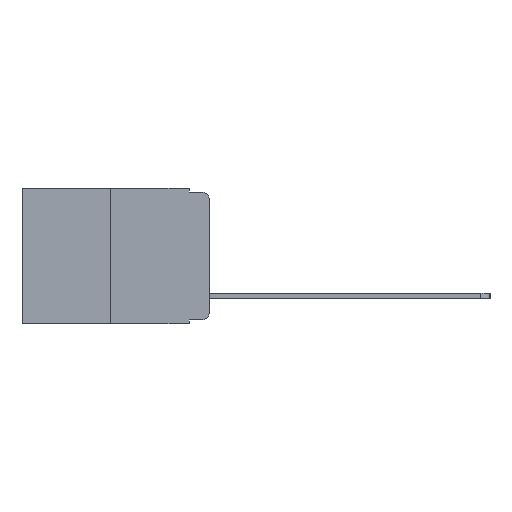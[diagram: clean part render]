
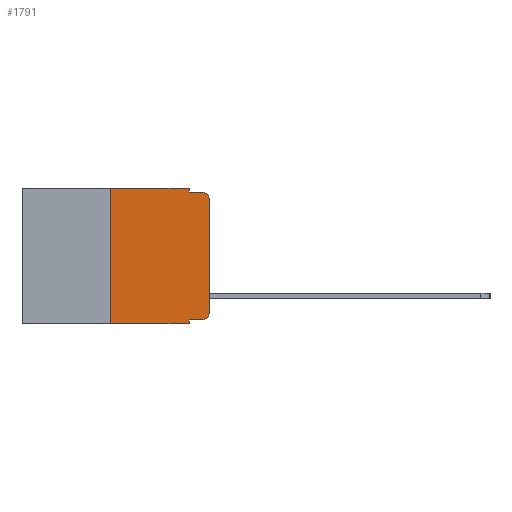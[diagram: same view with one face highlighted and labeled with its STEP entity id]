
A CAD part, left-side view. The second image highlights one B-rep face of the part: STEP entity #1791.
In plain terms, the highlighted planar face has unit normal (-1, 0, 0).
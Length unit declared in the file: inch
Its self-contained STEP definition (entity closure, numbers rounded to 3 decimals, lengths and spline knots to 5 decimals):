
#466 = ORIENTED_EDGE ( 'NONE', *, *, #8201, .T. ) ;
#548 = VERTEX_POINT ( 'NONE', #7839 ) ;
#556 = ORIENTED_EDGE ( 'NONE', *, *, #7493, .F. ) ;
#590 = EDGE_CURVE ( 'NONE', #3171, #14071, #6019, .T. ) ;
#1048 = DIRECTION ( 'NONE',  ( 0., 0., -1. ) ) ;
#1083 = CARTESIAN_POINT ( 'NONE',  ( 0., 0.25, 0. ) ) ;
#1155 = ORIENTED_EDGE ( 'NONE', *, *, #3099, .F. ) ;
#1208 = DIRECTION ( 'NONE',  ( 0., 0., -1. ) ) ;
#1324 = VERTEX_POINT ( 'NONE', #7119 ) ;
#1375 = CARTESIAN_POINT ( 'NONE',  ( 0., 0.02, -0.01 ) ) ;
#1388 = CIRCLE ( 'NONE', #4639, 0.02 ) ;
#1446 = EDGE_CURVE ( 'NONE', #3171, #1324, #8985, .T. ) ;
#1772 = ORIENTED_EDGE ( 'NONE', *, *, #1446, .F. ) ;
#1791 = ADVANCED_FACE ( 'NONE', ( #7825 ), #3639, .F. ) ;
#1793 = VECTOR ( 'NONE', #2860, 39.37008 ) ;
#1858 = LINE ( 'NONE', #7852, #13029 ) ;
#2022 = VECTOR ( 'NONE', #2295, 39.37008 ) ;
#2295 = DIRECTION ( 'NONE',  ( 0., -1., 0. ) ) ;
#2546 = ORIENTED_EDGE ( 'NONE', *, *, #590, .T. ) ;
#2860 = DIRECTION ( 'NONE',  ( 0., -1., 0. ) ) ;
#2901 = ORIENTED_EDGE ( 'NONE', *, *, #6678, .T. ) ;
#2930 = ORIENTED_EDGE ( 'NONE', *, *, #12642, .T. ) ;
#3069 = VECTOR ( 'NONE', #5308, 39.37008 ) ;
#3099 = EDGE_CURVE ( 'NONE', #548, #6558, #9092, .T. ) ;
#3103 = LINE ( 'NONE', #10808, #11281 ) ;
#3171 = VERTEX_POINT ( 'NONE', #7904 ) ;
#3335 = VERTEX_POINT ( 'NONE', #9480 ) ;
#3347 = VECTOR ( 'NONE', #12979, 39.37008 ) ;
#3639 = PLANE ( 'NONE',  #9066 ) ;
#3776 = CARTESIAN_POINT ( 'NONE',  ( 0., 0.051, 0. ) ) ;
#3792 = ORIENTED_EDGE ( 'NONE', *, *, #10269, .T. ) ;
#4016 = CARTESIAN_POINT ( 'NONE',  ( 0., 0.02, -0.313 ) ) ;
#4128 = AXIS2_PLACEMENT_3D ( 'NONE', #4016, #11450, #5133 ) ;
#4594 = EDGE_CURVE ( 'NONE', #11848, #3335, #11899, .T. ) ;
#4626 = DIRECTION ( 'NONE',  ( 0., 0., -1. ) ) ;
#4639 = AXIS2_PLACEMENT_3D ( 'NONE', #14218, #7967, #1208 ) ;
#4664 = CARTESIAN_POINT ( 'NONE',  ( 0., 0.473, 0. ) ) ;
#4993 = VERTEX_POINT ( 'NONE', #8993 ) ;
#5047 = LINE ( 'NONE', #6731, #2022 ) ;
#5054 = EDGE_LOOP ( 'NONE', ( #2901, #466, #556, #12918, #5198, #1155, #3792, #1772, #2546, #2930 ) ) ;
#5083 = VERTEX_POINT ( 'NONE', #5981 ) ;
#5133 = DIRECTION ( 'NONE',  ( 0., 0., -1. ) ) ;
#5198 = ORIENTED_EDGE ( 'NONE', *, *, #8661, .F. ) ;
#5308 = DIRECTION ( 'NONE',  ( 0., -1., 0. ) ) ;
#5480 = VECTOR ( 'NONE', #4626, 39.37008 ) ;
#5720 = VERTEX_POINT ( 'NONE', #1375 ) ;
#5731 = CARTESIAN_POINT ( 'NONE',  ( 0., 0.051, 0. ) ) ;
#5981 = CARTESIAN_POINT ( 'NONE',  ( 0., 0., -0.313 ) ) ;
#6019 = LINE ( 'NONE', #13628, #3069 ) ;
#6212 = CARTESIAN_POINT ( 'NONE',  ( 0., 0.02, -0.333 ) ) ;
#6558 = VERTEX_POINT ( 'NONE', #6598 ) ;
#6598 = CARTESIAN_POINT ( 'NONE',  ( 0., 0.25, 0. ) ) ;
#6660 = DIRECTION ( 'NONE',  ( 0., -1., 0. ) ) ;
#6678 = EDGE_CURVE ( 'NONE', #5083, #4993, #1858, .T. ) ;
#6731 = CARTESIAN_POINT ( 'NONE',  ( 0., 0.051, -0.01 ) ) ;
#7119 = CARTESIAN_POINT ( 'NONE',  ( 0., 0.051, -0.343 ) ) ;
#7245 = DIRECTION ( 'NONE',  ( 0., 0., -1. ) ) ;
#7493 = EDGE_CURVE ( 'NONE', #3335, #5720, #5047, .T. ) ;
#7726 = LINE ( 'NONE', #11367, #1793 ) ;
#7825 = FACE_OUTER_BOUND ( 'NONE', #5054, .T. ) ;
#7835 = DIRECTION ( 'NONE',  ( 1., 0., 0. ) ) ;
#7839 = CARTESIAN_POINT ( 'NONE',  ( 0., 0.25, -0.343 ) ) ;
#7852 = CARTESIAN_POINT ( 'NONE',  ( 0., 0., 0. ) ) ;
#7904 = CARTESIAN_POINT ( 'NONE',  ( 0., 0.051, -0.333 ) ) ;
#7967 = DIRECTION ( 'NONE',  ( -1., 0., 0. ) ) ;
#8201 = EDGE_CURVE ( 'NONE', #4993, #5720, #1388, .T. ) ;
#8619 = CIRCLE ( 'NONE', #4128, 0.02 ) ;
#8661 = EDGE_CURVE ( 'NONE', #6558, #11848, #3103, .T. ) ;
#8985 = LINE ( 'NONE', #3776, #5480 ) ;
#8993 = CARTESIAN_POINT ( 'NONE',  ( 0., 0., -0.03 ) ) ;
#9066 = AXIS2_PLACEMENT_3D ( 'NONE', #4664, #7835, #1048 ) ;
#9092 = LINE ( 'NONE', #1083, #3347 ) ;
#9140 = VECTOR ( 'NONE', #7245, 39.37008 ) ;
#9480 = CARTESIAN_POINT ( 'NONE',  ( 0., 0.051, -0.01 ) ) ;
#10269 = EDGE_CURVE ( 'NONE', #548, #1324, #7726, .T. ) ;
#10357 = CARTESIAN_POINT ( 'NONE',  ( 0., 0.051, 0. ) ) ;
#10808 = CARTESIAN_POINT ( 'NONE',  ( 0., 0.473, 0. ) ) ;
#11281 = VECTOR ( 'NONE', #6660, 39.37008 ) ;
#11367 = CARTESIAN_POINT ( 'NONE',  ( 0., 0.473, -0.343 ) ) ;
#11450 = DIRECTION ( 'NONE',  ( -1., 0., 0. ) ) ;
#11848 = VERTEX_POINT ( 'NONE', #5731 ) ;
#11899 = LINE ( 'NONE', #10357, #9140 ) ;
#12033 = DIRECTION ( 'NONE',  ( 0., 0., 1. ) ) ;
#12642 = EDGE_CURVE ( 'NONE', #14071, #5083, #8619, .T. ) ;
#12918 = ORIENTED_EDGE ( 'NONE', *, *, #4594, .F. ) ;
#12979 = DIRECTION ( 'NONE',  ( 0., 0., 1. ) ) ;
#13029 = VECTOR ( 'NONE', #12033, 39.37008 ) ;
#13628 = CARTESIAN_POINT ( 'NONE',  ( 0., 0.051, -0.333 ) ) ;
#14071 = VERTEX_POINT ( 'NONE', #6212 ) ;
#14218 = CARTESIAN_POINT ( 'NONE',  ( 0., 0.02, -0.03 ) ) ;
